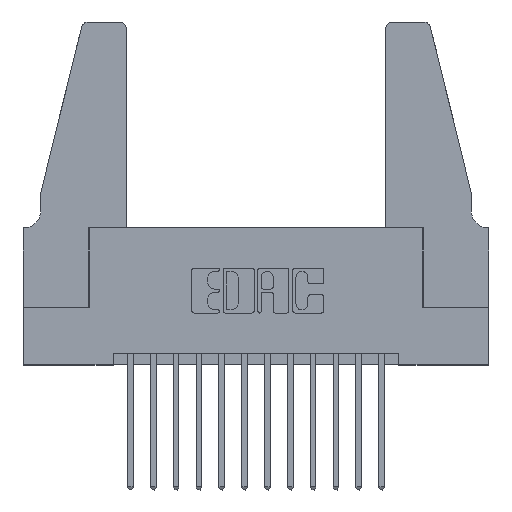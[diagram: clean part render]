
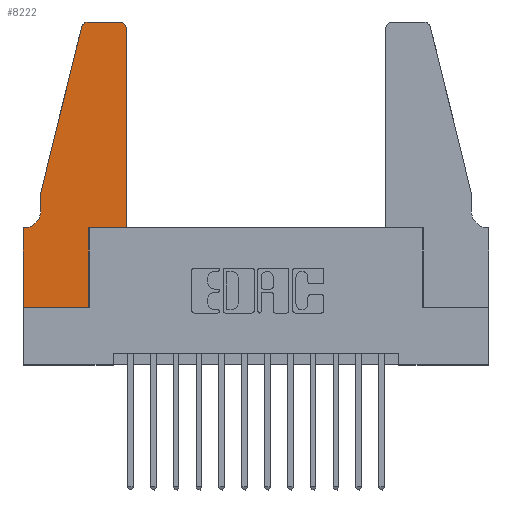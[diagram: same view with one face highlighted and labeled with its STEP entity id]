
A CAD part, top view. The second image highlights one B-rep face of the part: STEP entity #8222.
In plain terms, the highlighted planar face has unit normal (0, 0, 1).
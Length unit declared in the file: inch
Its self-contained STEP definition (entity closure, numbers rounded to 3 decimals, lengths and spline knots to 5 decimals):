
#86 = CARTESIAN_POINT ( 'NONE',  ( 0., 0.35, 0.37 ) ) ;
#383 = DIRECTION ( 'NONE',  ( 0., 0., 1. ) ) ;
#440 = EDGE_CURVE ( 'NONE', #3252, #3982, #15585, .T. ) ;
#443 = VECTOR ( 'NONE', #12755, 39.37008 ) ;
#770 = CARTESIAN_POINT ( 'NONE',  ( 0.0755, 0.35, 0.37 ) ) ;
#880 = LINE ( 'NONE', #4318, #13417 ) ;
#1002 = EDGE_CURVE ( 'NONE', #1056, #1705, #14097, .T. ) ;
#1056 = VERTEX_POINT ( 'NONE', #7290 ) ;
#1180 = ORIENTED_EDGE ( 'NONE', *, *, #12371, .T. ) ;
#1182 = ORIENTED_EDGE ( 'NONE', *, *, #6421, .T. ) ;
#1255 = ORIENTED_EDGE ( 'NONE', *, *, #10654, .T. ) ;
#1281 = CARTESIAN_POINT ( 'NONE',  ( 0.4505, 1.22, 0.37 ) ) ;
#1341 = CARTESIAN_POINT ( 'NONE',  ( 0., 0., 0.37 ) ) ;
#1363 = DIRECTION ( 'NONE',  ( 0., 1., 0. ) ) ;
#1503 = ORIENTED_EDGE ( 'NONE', *, *, #8481, .T. ) ;
#1577 = CARTESIAN_POINT ( 'NONE',  ( 0.25487, 1.22718, 0.37 ) ) ;
#1705 = VERTEX_POINT ( 'NONE', #4887 ) ;
#1728 = CARTESIAN_POINT ( 'NONE',  ( 0.0755, 0.5, 0.37 ) ) ;
#2577 = PLANE ( 'NONE',  #7054 ) ;
#2812 = VECTOR ( 'NONE', #1363, 39.37008 ) ;
#3082 = DIRECTION ( 'NONE',  ( 1., 0., 0. ) ) ;
#3252 = VERTEX_POINT ( 'NONE', #11917 ) ;
#3785 = VERTEX_POINT ( 'NONE', #1728 ) ;
#3930 = DIRECTION ( 'NONE',  ( 0., -1., 0. ) ) ;
#3982 = VERTEX_POINT ( 'NONE', #15305 ) ;
#4318 = CARTESIAN_POINT ( 'NONE',  ( 0.0755, 0.5, 0.37 ) ) ;
#4538 = CARTESIAN_POINT ( 'NONE',  ( 0.0055, 0.42, 0.37 ) ) ;
#4887 = CARTESIAN_POINT ( 'NONE',  ( 0.284, 1.25, 0.37 ) ) ;
#4889 = VERTEX_POINT ( 'NONE', #14876 ) ;
#5118 = DIRECTION ( 'NONE',  ( 1., 0., 0. ) ) ;
#5228 = EDGE_CURVE ( 'NONE', #7691, #3252, #14154, .T. ) ;
#5403 = CARTESIAN_POINT ( 'NONE',  ( 0.284, 1.22, 0.37 ) ) ;
#5603 = CARTESIAN_POINT ( 'NONE',  ( 0.4505, 0.35, 0.37 ) ) ;
#5625 = CARTESIAN_POINT ( 'NONE',  ( 0.0755, 0.5, 0.37 ) ) ;
#5648 = AXIS2_PLACEMENT_3D ( 'NONE', #5403, #13732, #6643 ) ;
#5672 = DIRECTION ( 'NONE',  ( 0., 1., 0. ) ) ;
#5785 = CARTESIAN_POINT ( 'NONE',  ( 0.2865, 0.35, 0.37 ) ) ;
#5823 = DIRECTION ( 'NONE',  ( -1., 0., 0. ) ) ;
#5968 = ORIENTED_EDGE ( 'NONE', *, *, #13940, .T. ) ;
#6076 = VERTEX_POINT ( 'NONE', #14546 ) ;
#6089 = VERTEX_POINT ( 'NONE', #1281 ) ;
#6421 = EDGE_CURVE ( 'NONE', #3785, #13157, #880, .T. ) ;
#6643 = DIRECTION ( 'NONE',  ( 1., 0., 0. ) ) ;
#6649 = LINE ( 'NONE', #11172, #10197 ) ;
#6743 = VECTOR ( 'NONE', #5672, 39.37008 ) ;
#6903 = CIRCLE ( 'NONE', #15333, 0.03 ) ;
#7054 = AXIS2_PLACEMENT_3D ( 'NONE', #86, #12271, #5118 ) ;
#7141 = ORIENTED_EDGE ( 'NONE', *, *, #11900, .T. ) ;
#7150 = EDGE_CURVE ( 'NONE', #6089, #1056, #6903, .T. ) ;
#7290 = CARTESIAN_POINT ( 'NONE',  ( 0.4205, 1.25, 0.37 ) ) ;
#7426 = VECTOR ( 'NONE', #9049, 39.37008 ) ;
#7649 = VECTOR ( 'NONE', #10566, 39.37008 ) ;
#7691 = VERTEX_POINT ( 'NONE', #1341 ) ;
#7796 = CARTESIAN_POINT ( 'NONE',  ( 0.4205, 1.22, 0.37 ) ) ;
#7834 = EDGE_CURVE ( 'NONE', #9026, #3785, #9851, .T. ) ;
#7853 = ORIENTED_EDGE ( 'NONE', *, *, #15436, .T. ) ;
#8043 = ORIENTED_EDGE ( 'NONE', *, *, #5228, .T. ) ;
#8222 = ADVANCED_FACE ( 'NONE', ( #11320 ), #2577, .T. ) ;
#8395 = DIRECTION ( 'NONE',  ( 1., 0., 0. ) ) ;
#8481 = EDGE_CURVE ( 'NONE', #3982, #6076, #13163, .T. ) ;
#9001 = CARTESIAN_POINT ( 'NONE',  ( 0.2605, 1.25, 0.37 ) ) ;
#9006 = DIRECTION ( 'NONE',  ( 1., 0., 0. ) ) ;
#9026 = VERTEX_POINT ( 'NONE', #1577 ) ;
#9049 = DIRECTION ( 'NONE',  ( -1., 0., 0. ) ) ;
#9340 = ORIENTED_EDGE ( 'NONE', *, *, #7834, .T. ) ;
#9396 = EDGE_LOOP ( 'NONE', ( #11982, #1180, #9340, #1182, #7853, #7141, #5968, #8043, #13833, #1503, #1255, #11492 ) ) ;
#9546 = LINE ( 'NONE', #12800, #6743 ) ;
#9851 = LINE ( 'NONE', #5625, #443 ) ;
#10197 = VECTOR ( 'NONE', #3930, 39.37008 ) ;
#10566 = DIRECTION ( 'NONE',  ( -1., 0., 0. ) ) ;
#10654 = EDGE_CURVE ( 'NONE', #6076, #6089, #9546, .T. ) ;
#10923 = CIRCLE ( 'NONE', #13057, 0.07 ) ;
#11027 = VECTOR ( 'NONE', #8395, 39.37008 ) ;
#11172 = CARTESIAN_POINT ( 'NONE',  ( 0., 0., 0.37 ) ) ;
#11320 = FACE_OUTER_BOUND ( 'NONE', #9396, .T. ) ;
#11492 = ORIENTED_EDGE ( 'NONE', *, *, #7150, .T. ) ;
#11715 = VERTEX_POINT ( 'NONE', #14878 ) ;
#11900 = EDGE_CURVE ( 'NONE', #11715, #4889, #13941, .T. ) ;
#11917 = CARTESIAN_POINT ( 'NONE',  ( 0.2865, 0., 0.37 ) ) ;
#11982 = ORIENTED_EDGE ( 'NONE', *, *, #1002, .T. ) ;
#12271 = DIRECTION ( 'NONE',  ( 0., 0., 1. ) ) ;
#12371 = EDGE_CURVE ( 'NONE', #1705, #9026, #13925, .T. ) ;
#12755 = DIRECTION ( 'NONE',  ( -0.239, -0.971, 0. ) ) ;
#12775 = VECTOR ( 'NONE', #3082, 39.37008 ) ;
#12800 = CARTESIAN_POINT ( 'NONE',  ( 0.4505, 0.35, 0.37 ) ) ;
#12940 = DIRECTION ( 'NONE',  ( 0., 0., -1. ) ) ;
#13057 = AXIS2_PLACEMENT_3D ( 'NONE', #4538, #12940, #5823 ) ;
#13157 = VERTEX_POINT ( 'NONE', #14394 ) ;
#13163 = LINE ( 'NONE', #5603, #12775 ) ;
#13417 = VECTOR ( 'NONE', #15090, 39.37008 ) ;
#13732 = DIRECTION ( 'NONE',  ( 0., 0., 1. ) ) ;
#13833 = ORIENTED_EDGE ( 'NONE', *, *, #440, .T. ) ;
#13925 = CIRCLE ( 'NONE', #5648, 0.03 ) ;
#13940 = EDGE_CURVE ( 'NONE', #4889, #7691, #6649, .T. ) ;
#13941 = LINE ( 'NONE', #770, #7649 ) ;
#14097 = LINE ( 'NONE', #9001, #7426 ) ;
#14154 = LINE ( 'NONE', #15437, #11027 ) ;
#14394 = CARTESIAN_POINT ( 'NONE',  ( 0.0755, 0.42, 0.37 ) ) ;
#14546 = CARTESIAN_POINT ( 'NONE',  ( 0.4505, 0.35, 0.37 ) ) ;
#14876 = CARTESIAN_POINT ( 'NONE',  ( 0., 0.35, 0.37 ) ) ;
#14878 = CARTESIAN_POINT ( 'NONE',  ( 0.0055, 0.35, 0.37 ) ) ;
#15090 = DIRECTION ( 'NONE',  ( 0., -1., 0. ) ) ;
#15305 = CARTESIAN_POINT ( 'NONE',  ( 0.2865, 0.35, 0.37 ) ) ;
#15333 = AXIS2_PLACEMENT_3D ( 'NONE', #7796, #383, #9006 ) ;
#15436 = EDGE_CURVE ( 'NONE', #13157, #11715, #10923, .T. ) ;
#15437 = CARTESIAN_POINT ( 'NONE',  ( 0., 0., 0.37 ) ) ;
#15585 = LINE ( 'NONE', #5785, #2812 ) ;
